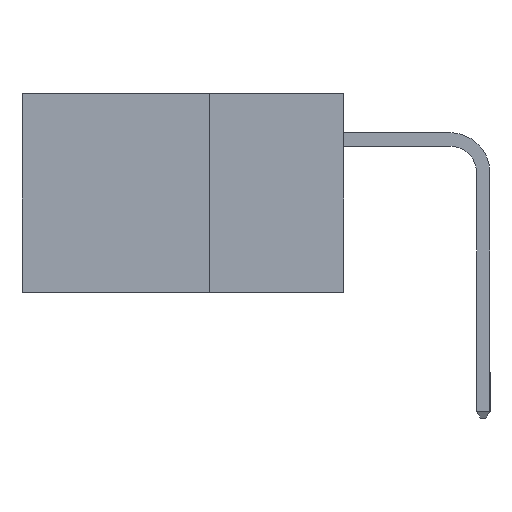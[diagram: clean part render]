
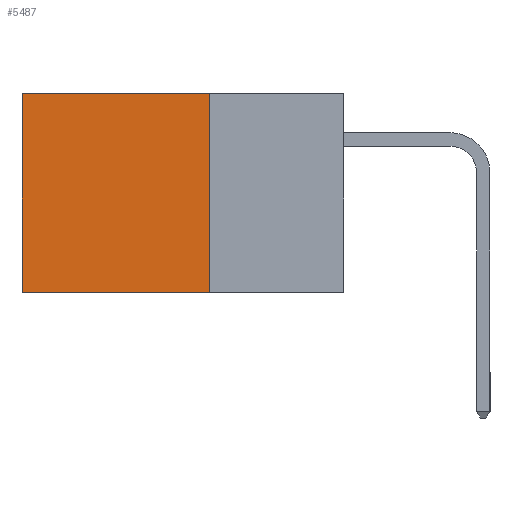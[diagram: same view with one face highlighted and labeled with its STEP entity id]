
A CAD part, left-side view. The second image highlights one B-rep face of the part: STEP entity #5487.
In plain terms, the highlighted planar face has unit normal (-1, 0, 0).
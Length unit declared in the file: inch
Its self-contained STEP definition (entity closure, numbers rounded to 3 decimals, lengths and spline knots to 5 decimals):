
#498 = DIRECTION ( 'NONE',  ( 0., 0., -1. ) ) ;
#944 = VERTEX_POINT ( 'NONE', #2296 ) ;
#1590 = LINE ( 'NONE', #14047, #9531 ) ;
#1848 = CARTESIAN_POINT ( 'NONE',  ( 0.298, 0.6, -0.37 ) ) ;
#1952 = DIRECTION ( 'NONE',  ( 0., 0., -1. ) ) ;
#2296 = CARTESIAN_POINT ( 'NONE',  ( 0.298, 0.6, 0. ) ) ;
#2758 = ORIENTED_EDGE ( 'NONE', *, *, #11943, .T. ) ;
#3048 = DIRECTION ( 'NONE',  ( 1., 0., 0. ) ) ;
#3185 = PLANE ( 'NONE',  #11709 ) ;
#3486 = CARTESIAN_POINT ( 'NONE',  ( 0.298, 0.25, 0. ) ) ;
#3803 = EDGE_CURVE ( 'NONE', #7407, #944, #1590, .T. ) ;
#3977 = EDGE_CURVE ( 'NONE', #11687, #7175, #6147, .T. ) ;
#4656 = CARTESIAN_POINT ( 'NONE',  ( 0.298, 0.25, -0.37 ) ) ;
#5431 = ORIENTED_EDGE ( 'NONE', *, *, #3977, .F. ) ;
#5487 = ADVANCED_FACE ( 'NONE', ( #13678 ), #3185, .F. ) ;
#5762 = EDGE_CURVE ( 'NONE', #7407, #11687, #8677, .T. ) ;
#6077 = LINE ( 'NONE', #6469, #14102 ) ;
#6088 = ORIENTED_EDGE ( 'NONE', *, *, #5762, .F. ) ;
#6147 = LINE ( 'NONE', #7189, #8094 ) ;
#6469 = CARTESIAN_POINT ( 'NONE',  ( 0.298, 0.6, 0. ) ) ;
#7175 = VERTEX_POINT ( 'NONE', #1848 ) ;
#7189 = CARTESIAN_POINT ( 'NONE',  ( 0.298, 0.25, -0.37 ) ) ;
#7407 = VERTEX_POINT ( 'NONE', #3486 ) ;
#8094 = VECTOR ( 'NONE', #9474, 39.37008 ) ;
#8341 = EDGE_LOOP ( 'NONE', ( #2758, #5431, #6088, #11552 ) ) ;
#8677 = LINE ( 'NONE', #13979, #10268 ) ;
#8743 = CARTESIAN_POINT ( 'NONE',  ( 0.298, 0.25, 0. ) ) ;
#9474 = DIRECTION ( 'NONE',  ( 0., 1., 0. ) ) ;
#9531 = VECTOR ( 'NONE', #13954, 39.37008 ) ;
#10268 = VECTOR ( 'NONE', #498, 39.37008 ) ;
#11552 = ORIENTED_EDGE ( 'NONE', *, *, #3803, .T. ) ;
#11687 = VERTEX_POINT ( 'NONE', #4656 ) ;
#11709 = AXIS2_PLACEMENT_3D ( 'NONE', #8743, #3048, #12085 ) ;
#11943 = EDGE_CURVE ( 'NONE', #944, #7175, #6077, .T. ) ;
#12085 = DIRECTION ( 'NONE',  ( 0., 0., -1. ) ) ;
#13678 = FACE_OUTER_BOUND ( 'NONE', #8341, .T. ) ;
#13954 = DIRECTION ( 'NONE',  ( 0., 1., 0. ) ) ;
#13979 = CARTESIAN_POINT ( 'NONE',  ( 0.298, 0.25, 0. ) ) ;
#14047 = CARTESIAN_POINT ( 'NONE',  ( 0.298, 0.25, 0. ) ) ;
#14102 = VECTOR ( 'NONE', #1952, 39.37008 ) ;
